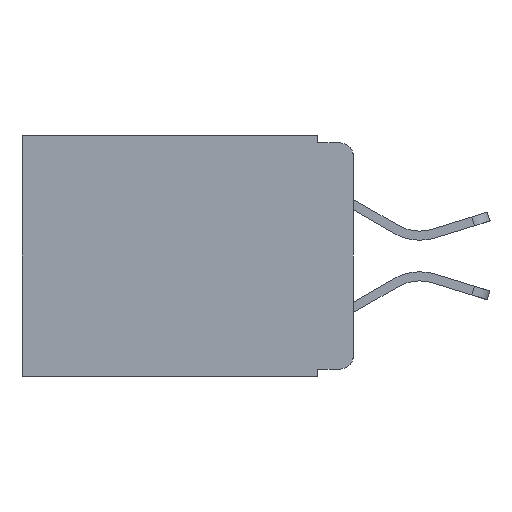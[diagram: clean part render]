
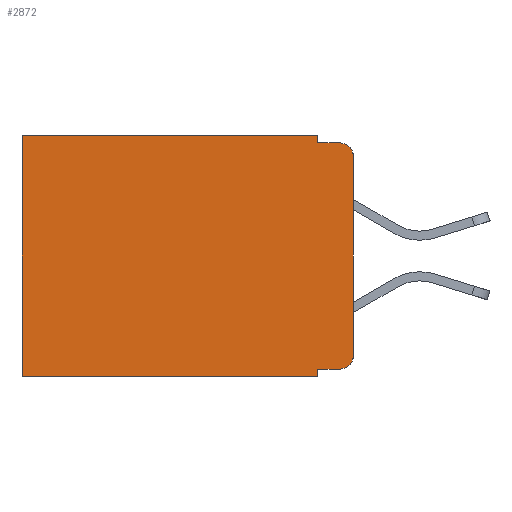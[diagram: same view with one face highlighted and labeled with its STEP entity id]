
A CAD part, left-side view. The second image highlights one B-rep face of the part: STEP entity #2872.
In plain terms, the highlighted planar face has unit normal (-1, 0, 0).
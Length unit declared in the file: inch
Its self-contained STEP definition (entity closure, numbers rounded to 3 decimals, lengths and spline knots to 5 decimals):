
#59 = EDGE_LOOP ( 'NONE', ( #12332, #4125, #3893, #3064, #3139, #3247, #3392, #3365, #3482, #3421 ) ) ;
#264 = VECTOR ( 'NONE', #765, 39.37008 ) ;
#390 = AXIS2_PLACEMENT_3D ( 'NONE', #10595, #2114, #10676 ) ;
#715 = VERTEX_POINT ( 'NONE', #11124 ) ;
#765 = DIRECTION ( 'NONE',  ( 0., 0., -1. ) ) ;
#810 = VECTOR ( 'NONE', #8511, 39.37008 ) ;
#951 = LINE ( 'NONE', #2685, #7258 ) ;
#1146 = VERTEX_POINT ( 'NONE', #3763 ) ;
#2110 = VECTOR ( 'NONE', #6038, 39.37008 ) ;
#2112 = CARTESIAN_POINT ( 'NONE',  ( 0.298, 0., -0.313 ) ) ;
#2114 = DIRECTION ( 'NONE',  ( 1., 0., 0. ) ) ;
#2183 = EDGE_CURVE ( 'NONE', #5086, #715, #5547, .T. ) ;
#2273 = VERTEX_POINT ( 'NONE', #6369 ) ;
#2685 = CARTESIAN_POINT ( 'NONE',  ( 0.298, 0., 0. ) ) ;
#2872 = ADVANCED_FACE ( 'NONE', ( #4236 ), #10540, .F. ) ;
#2990 = EDGE_CURVE ( 'NONE', #6016, #6164, #13052, .T. ) ;
#3064 = ORIENTED_EDGE ( 'NONE', *, *, #2990, .F. ) ;
#3139 = ORIENTED_EDGE ( 'NONE', *, *, #5107, .T. ) ;
#3247 = ORIENTED_EDGE ( 'NONE', *, *, #8955, .T. ) ;
#3365 = ORIENTED_EDGE ( 'NONE', *, *, #6166, .F. ) ;
#3392 = ORIENTED_EDGE ( 'NONE', *, *, #12508, .F. ) ;
#3421 = ORIENTED_EDGE ( 'NONE', *, *, #6882, .T. ) ;
#3482 = ORIENTED_EDGE ( 'NONE', *, *, #9127, .T. ) ;
#3548 = LINE ( 'NONE', #13404, #264 ) ;
#3759 = DIRECTION ( 'NONE',  ( -1., 0., 0. ) ) ;
#3763 = CARTESIAN_POINT ( 'NONE',  ( 0.298, 0.051, -0.333 ) ) ;
#3886 = AXIS2_PLACEMENT_3D ( 'NONE', #7232, #7207, #11906 ) ;
#3893 = ORIENTED_EDGE ( 'NONE', *, *, #4614, .F. ) ;
#3916 = DIRECTION ( 'NONE',  ( 0., 0., -1. ) ) ;
#4120 = VECTOR ( 'NONE', #6966, 39.37008 ) ;
#4125 = ORIENTED_EDGE ( 'NONE', *, *, #2183, .T. ) ;
#4236 = FACE_OUTER_BOUND ( 'NONE', #59, .T. ) ;
#4373 = CARTESIAN_POINT ( 'NONE',  ( 0.298, 0.051, -0.343 ) ) ;
#4414 = LINE ( 'NONE', #13168, #810 ) ;
#4614 = EDGE_CURVE ( 'NONE', #6164, #715, #6252, .T. ) ;
#4622 = CARTESIAN_POINT ( 'NONE',  ( 0.298, 0.02, -0.333 ) ) ;
#4858 = DIRECTION ( 'NONE',  ( 0., -1., 0. ) ) ;
#4882 = CARTESIAN_POINT ( 'NONE',  ( 0.298, 0., -0.343 ) ) ;
#5086 = VERTEX_POINT ( 'NONE', #5242 ) ;
#5107 = EDGE_CURVE ( 'NONE', #6016, #2273, #4414, .T. ) ;
#5242 = CARTESIAN_POINT ( 'NONE',  ( 0.298, 0., -0.03 ) ) ;
#5546 = VECTOR ( 'NONE', #4858, 39.37008 ) ;
#5547 = CIRCLE ( 'NONE', #3886, 0.02 ) ;
#5822 = VERTEX_POINT ( 'NONE', #4622 ) ;
#6016 = VERTEX_POINT ( 'NONE', #8202 ) ;
#6038 = DIRECTION ( 'NONE',  ( 0., 1., 0. ) ) ;
#6164 = VERTEX_POINT ( 'NONE', #8979 ) ;
#6166 = EDGE_CURVE ( 'NONE', #1146, #8940, #9843, .T. ) ;
#6252 = LINE ( 'NONE', #10488, #5546 ) ;
#6369 = CARTESIAN_POINT ( 'NONE',  ( 0.298, 0.473, 0. ) ) ;
#6882 = EDGE_CURVE ( 'NONE', #5822, #13584, #8184, .T. ) ;
#6918 = CARTESIAN_POINT ( 'NONE',  ( 0.298, 0.051, -0.333 ) ) ;
#6945 = EDGE_CURVE ( 'NONE', #5086, #13584, #951, .T. ) ;
#6966 = DIRECTION ( 'NONE',  ( 0., -1., 0. ) ) ;
#7207 = DIRECTION ( 'NONE',  ( -1., 0., 0. ) ) ;
#7211 = LINE ( 'NONE', #6918, #4120 ) ;
#7232 = CARTESIAN_POINT ( 'NONE',  ( 0.298, 0.02, -0.03 ) ) ;
#7258 = VECTOR ( 'NONE', #3916, 39.37008 ) ;
#7783 = AXIS2_PLACEMENT_3D ( 'NONE', #10135, #3759, #11056 ) ;
#8184 = CIRCLE ( 'NONE', #7783, 0.02 ) ;
#8202 = CARTESIAN_POINT ( 'NONE',  ( 0.298, 0.051, 0. ) ) ;
#8511 = DIRECTION ( 'NONE',  ( 0., 1., 0. ) ) ;
#8612 = DIRECTION ( 'NONE',  ( 0., 0., -1. ) ) ;
#8830 = CARTESIAN_POINT ( 'NONE',  ( 0.298, 0.051, 0. ) ) ;
#8940 = VERTEX_POINT ( 'NONE', #4373 ) ;
#8955 = EDGE_CURVE ( 'NONE', #2273, #11926, #3548, .T. ) ;
#8979 = CARTESIAN_POINT ( 'NONE',  ( 0.298, 0.051, -0.01 ) ) ;
#9023 = DIRECTION ( 'NONE',  ( 0., 0., -1. ) ) ;
#9127 = EDGE_CURVE ( 'NONE', #1146, #5822, #7211, .T. ) ;
#9843 = LINE ( 'NONE', #8830, #12009 ) ;
#10135 = CARTESIAN_POINT ( 'NONE',  ( 0.298, 0.02, -0.313 ) ) ;
#10255 = CARTESIAN_POINT ( 'NONE',  ( 0.298, 0.051, 0. ) ) ;
#10488 = CARTESIAN_POINT ( 'NONE',  ( 0.298, 0.051, -0.01 ) ) ;
#10540 = PLANE ( 'NONE',  #390 ) ;
#10595 = CARTESIAN_POINT ( 'NONE',  ( 0.298, 0., 0. ) ) ;
#10676 = DIRECTION ( 'NONE',  ( 0., 0., -1. ) ) ;
#10719 = LINE ( 'NONE', #4882, #2110 ) ;
#11056 = DIRECTION ( 'NONE',  ( 0., 0., -1. ) ) ;
#11124 = CARTESIAN_POINT ( 'NONE',  ( 0.298, 0.02, -0.01 ) ) ;
#11169 = VECTOR ( 'NONE', #8612, 39.37008 ) ;
#11906 = DIRECTION ( 'NONE',  ( 0., 0., -1. ) ) ;
#11926 = VERTEX_POINT ( 'NONE', #12125 ) ;
#12009 = VECTOR ( 'NONE', #9023, 39.37008 ) ;
#12125 = CARTESIAN_POINT ( 'NONE',  ( 0.298, 0.473, -0.343 ) ) ;
#12332 = ORIENTED_EDGE ( 'NONE', *, *, #6945, .F. ) ;
#12508 = EDGE_CURVE ( 'NONE', #8940, #11926, #10719, .T. ) ;
#13052 = LINE ( 'NONE', #10255, #11169 ) ;
#13168 = CARTESIAN_POINT ( 'NONE',  ( 0.298, 0., 0. ) ) ;
#13404 = CARTESIAN_POINT ( 'NONE',  ( 0.298, 0.473, 0. ) ) ;
#13584 = VERTEX_POINT ( 'NONE', #2112 ) ;
